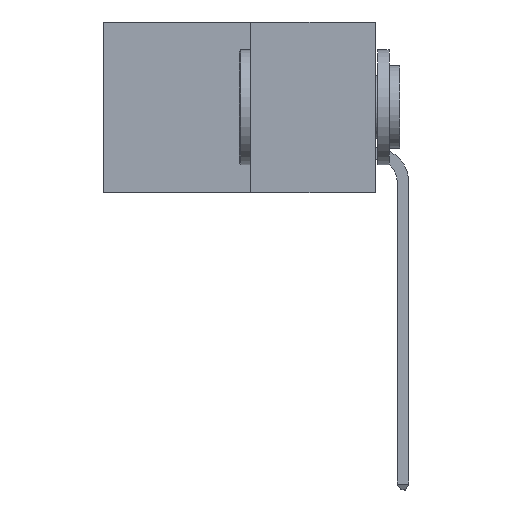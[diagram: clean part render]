
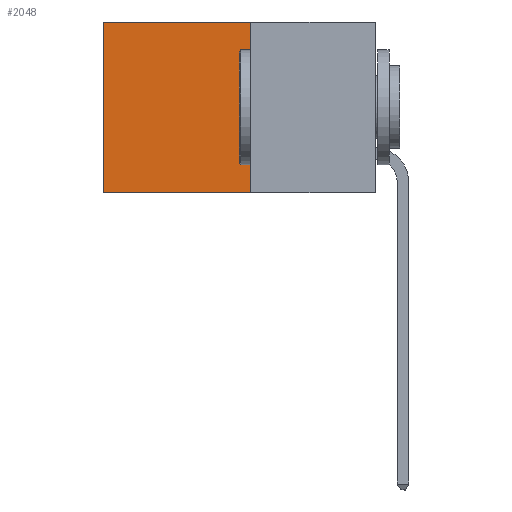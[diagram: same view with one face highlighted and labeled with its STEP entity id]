
A CAD part, left-side view. The second image highlights one B-rep face of the part: STEP entity #2048.
In plain terms, the highlighted planar face has unit normal (-1, 0, 0).
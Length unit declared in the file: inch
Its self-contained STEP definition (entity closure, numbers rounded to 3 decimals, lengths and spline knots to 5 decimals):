
#355 = DIRECTION ( 'NONE',  ( 0., 0., -1. ) ) ;
#523 = EDGE_CURVE ( 'NONE', #9756, #2715, #2932, .T. ) ;
#610 = ORIENTED_EDGE ( 'NONE', *, *, #523, .F. ) ;
#1043 = CARTESIAN_POINT ( 'NONE',  ( 0.277, 0.59, 0. ) ) ;
#1163 = ORIENTED_EDGE ( 'NONE', *, *, #13693, .F. ) ;
#1228 = CARTESIAN_POINT ( 'NONE',  ( 0.277, 0.27, -0.37 ) ) ;
#1416 = EDGE_LOOP ( 'NONE', ( #10645, #1163, #610, #2029 ) ) ;
#2029 = ORIENTED_EDGE ( 'NONE', *, *, #13587, .T. ) ;
#2048 = ADVANCED_FACE ( 'NONE', ( #11470 ), #3530, .F. ) ;
#2354 = DIRECTION ( 'NONE',  ( 0., 1., 0. ) ) ;
#2533 = EDGE_CURVE ( 'NONE', #10638, #8409, #5370, .T. ) ;
#2715 = VERTEX_POINT ( 'NONE', #8739 ) ;
#2932 = LINE ( 'NONE', #6901, #5254 ) ;
#3132 = CARTESIAN_POINT ( 'NONE',  ( 0.277, 0.59, -0.37 ) ) ;
#3530 = PLANE ( 'NONE',  #13835 ) ;
#4632 = LINE ( 'NONE', #14086, #10737 ) ;
#4935 = CARTESIAN_POINT ( 'NONE',  ( 0.277, 0.59, -0.37 ) ) ;
#5003 = VECTOR ( 'NONE', #355, 39.37008 ) ;
#5098 = DIRECTION ( 'NONE',  ( 0., 0., -1. ) ) ;
#5254 = VECTOR ( 'NONE', #9363, 39.37008 ) ;
#5370 = LINE ( 'NONE', #4935, #5003 ) ;
#5889 = VECTOR ( 'NONE', #2354, 39.37008 ) ;
#6181 = DIRECTION ( 'NONE',  ( 0., 1., 0. ) ) ;
#6399 = CARTESIAN_POINT ( 'NONE',  ( 0.277, 0.27, -0.37 ) ) ;
#6901 = CARTESIAN_POINT ( 'NONE',  ( 0.277, 0.27, -0.37 ) ) ;
#8409 = VERTEX_POINT ( 'NONE', #3132 ) ;
#8739 = CARTESIAN_POINT ( 'NONE',  ( 0.277, 0.27, -0.37 ) ) ;
#9363 = DIRECTION ( 'NONE',  ( 0., 0., -1. ) ) ;
#9756 = VERTEX_POINT ( 'NONE', #10391 ) ;
#10391 = CARTESIAN_POINT ( 'NONE',  ( 0.277, 0.27, 0. ) ) ;
#10638 = VERTEX_POINT ( 'NONE', #1043 ) ;
#10645 = ORIENTED_EDGE ( 'NONE', *, *, #2533, .T. ) ;
#10737 = VECTOR ( 'NONE', #6181, 39.37008 ) ;
#11244 = DIRECTION ( 'NONE',  ( 1., 0., 0. ) ) ;
#11470 = FACE_OUTER_BOUND ( 'NONE', #1416, .T. ) ;
#11956 = LINE ( 'NONE', #1228, #5889 ) ;
#13587 = EDGE_CURVE ( 'NONE', #9756, #10638, #4632, .T. ) ;
#13693 = EDGE_CURVE ( 'NONE', #2715, #8409, #11956, .T. ) ;
#13835 = AXIS2_PLACEMENT_3D ( 'NONE', #6399, #11244, #5098 ) ;
#14086 = CARTESIAN_POINT ( 'NONE',  ( 0.277, 0.27, 0. ) ) ;
